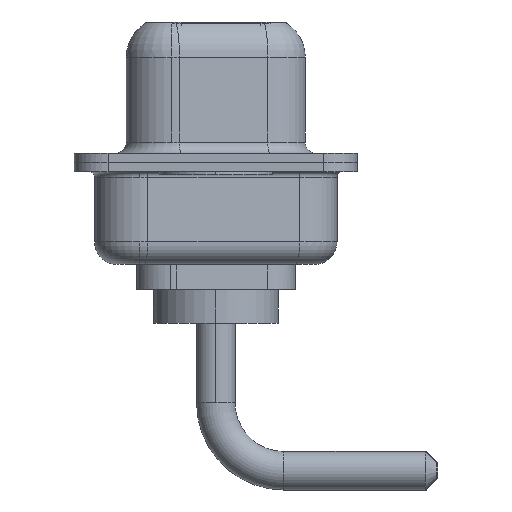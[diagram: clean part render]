
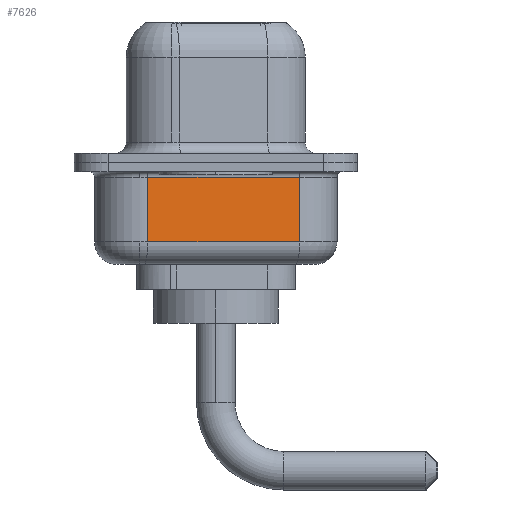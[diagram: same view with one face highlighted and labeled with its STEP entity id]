
A CAD part, left-side view. The second image highlights one B-rep face of the part: STEP entity #7626.
In plain terms, the highlighted planar face has unit normal (-0.985, -0.174, 0).
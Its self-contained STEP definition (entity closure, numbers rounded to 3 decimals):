
#275 = VECTOR ( 'NONE', #6946, 1000. ) ;
#307 = ORIENTED_EDGE ( 'NONE', *, *, #3711, .T. ) ;
#430 = LINE ( 'NONE', #9350, #5089 ) ;
#843 = CARTESIAN_POINT ( 'NONE',  ( 4.062, -3.697, -0.65 ) ) ;
#1577 = LINE ( 'NONE', #10479, #6525 ) ;
#1933 = CARTESIAN_POINT ( 'NONE',  ( 2.88, 3.003, -0.65 ) ) ;
#2587 = PLANE ( 'NONE',  #4350 ) ;
#3170 = VERTEX_POINT ( 'NONE', #5655 ) ;
#3381 = DIRECTION ( 'NONE',  ( 0.174, -0.985, 0. ) ) ;
#3555 = DIRECTION ( 'NONE',  ( -0.174, 0.985, 0. ) ) ;
#3711 = EDGE_CURVE ( 'NONE', #3170, #8389, #430, .T. ) ;
#3752 = CARTESIAN_POINT ( 'NONE',  ( 2.88, 3.003, -0.65 ) ) ;
#4208 = VECTOR ( 'NONE', #10035, 1000. ) ;
#4350 = AXIS2_PLACEMENT_3D ( 'NONE', #7965, #6230, #3555 ) ;
#4778 = EDGE_CURVE ( 'NONE', #11043, #3170, #1577, .T. ) ;
#5089 = VECTOR ( 'NONE', #8390, 1000. ) ;
#5655 = CARTESIAN_POINT ( 'NONE',  ( 4.062, -3.697, -3.5 ) ) ;
#6038 = CARTESIAN_POINT ( 'NONE',  ( 2.88, 3.003, -3.5 ) ) ;
#6230 = DIRECTION ( 'NONE',  ( 0.985, 0.174, 0. ) ) ;
#6525 = VECTOR ( 'NONE', #3381, 1000. ) ;
#6540 = EDGE_LOOP ( 'NONE', ( #10739, #7798, #307, #10122 ) ) ;
#6849 = EDGE_CURVE ( 'NONE', #11043, #9499, #7816, .T. ) ;
#6946 = DIRECTION ( 'NONE',  ( 0., 0., 1. ) ) ;
#7626 = ADVANCED_FACE ( 'NONE', ( #10548 ), #2587, .F. ) ;
#7798 = ORIENTED_EDGE ( 'NONE', *, *, #4778, .T. ) ;
#7816 = LINE ( 'NONE', #8526, #275 ) ;
#7965 = CARTESIAN_POINT ( 'NONE',  ( 2.88, 3.003, -4.5 ) ) ;
#8389 = VERTEX_POINT ( 'NONE', #843 ) ;
#8390 = DIRECTION ( 'NONE',  ( 0., 0., 1. ) ) ;
#8526 = CARTESIAN_POINT ( 'NONE',  ( 2.88, 3.003, -4.5 ) ) ;
#8970 = LINE ( 'NONE', #1933, #4208 ) ;
#9350 = CARTESIAN_POINT ( 'NONE',  ( 4.062, -3.697, -4.5 ) ) ;
#9499 = VERTEX_POINT ( 'NONE', #3752 ) ;
#10035 = DIRECTION ( 'NONE',  ( -0.174, 0.985, 0. ) ) ;
#10122 = ORIENTED_EDGE ( 'NONE', *, *, #10247, .T. ) ;
#10247 = EDGE_CURVE ( 'NONE', #8389, #9499, #8970, .T. ) ;
#10479 = CARTESIAN_POINT ( 'NONE',  ( 2.88, 3.003, -3.5 ) ) ;
#10548 = FACE_OUTER_BOUND ( 'NONE', #6540, .T. ) ;
#10739 = ORIENTED_EDGE ( 'NONE', *, *, #6849, .F. ) ;
#11043 = VERTEX_POINT ( 'NONE', #6038 ) ;
